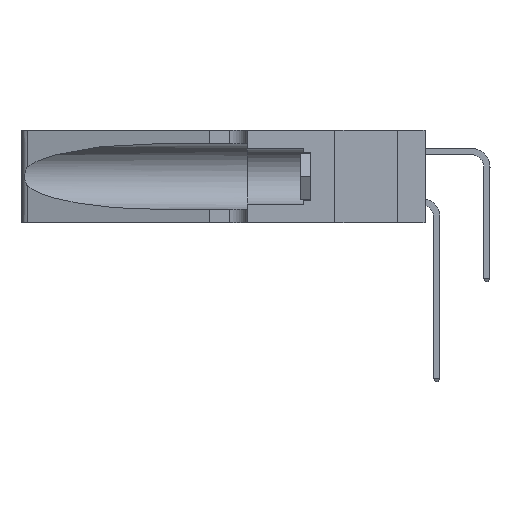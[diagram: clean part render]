
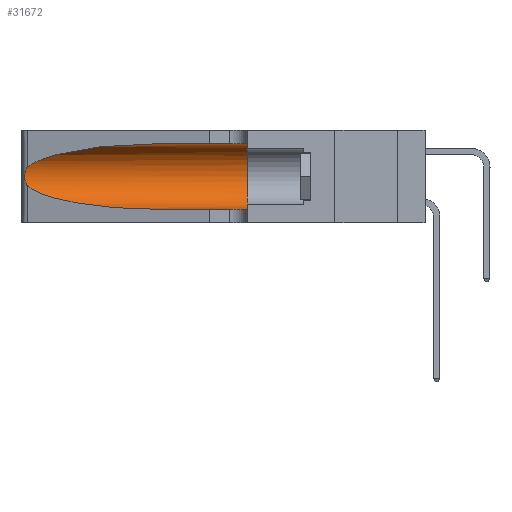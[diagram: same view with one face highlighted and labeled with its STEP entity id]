
A CAD part, left-side view. The second image highlights one B-rep face of the part: STEP entity #31672.
In plain terms, the highlighted cylindrical face has radius 3.308 mm (diameter 6.617 mm), a partial arc.
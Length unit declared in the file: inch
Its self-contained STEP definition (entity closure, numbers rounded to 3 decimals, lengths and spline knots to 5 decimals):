
#362 = CARTESIAN_POINT ( 'NONE',  ( 0.26017, 1.23833, 0.17102 ) ) ;
#567 = EDGE_LOOP ( 'NONE', ( #5458, #7572, #2621, #29499, #17899, #40339 ) ) ;
#2184 = CARTESIAN_POINT ( 'NONE',  ( 0.1305, 1.61858, 0.31525 ) ) ;
#2621 = ORIENTED_EDGE ( 'NONE', *, *, #37447, .T. ) ;
#4915 = CARTESIAN_POINT ( 'NONE',  ( 0.2373, 1.15595, 0.08982 ) ) ;
#5210 = CARTESIAN_POINT ( 'NONE',  ( 0.25487, 1.22718, 0.22369 ) ) ;
#5458 = ORIENTED_EDGE ( 'NONE', *, *, #31638, .T. ) ;
#5500 = CARTESIAN_POINT ( 'NONE',  ( 0.25555, 1.22994, 0.2215 ) ) ;
#5758 = CARTESIAN_POINT ( 'NONE',  ( 0.1305, 0.72297, 0.05475 ) ) ;
#5780 = CARTESIAN_POINT ( 'NONE',  ( 0.25487, 1.22718, 0.14631 ) ) ;
#6291 = VERTEX_POINT ( 'NONE', #24613 ) ;
#6397 = VERTEX_POINT ( 'NONE', #15946 ) ;
#7291 = CARTESIAN_POINT ( 'NONE',  ( 0.25487, 1.22718, 0.22369 ) ) ;
#7572 = ORIENTED_EDGE ( 'NONE', *, *, #22277, .T. ) ;
#8047 = DIRECTION ( 'NONE',  ( 0., -1., 0. ) ) ;
#8286 = DIRECTION ( 'NONE',  ( 0., 0., 1. ) ) ;
#8393 = CARTESIAN_POINT ( 'NONE',  ( 0.1305, 0.72297, 0.05475 ) ) ;
#8981 = CARTESIAN_POINT ( 'NONE',  ( 0.25854, 1.2359, 0.20912 ) ) ;
#10666 = CARTESIAN_POINT ( 'NONE',  ( 0.1305, 1.61858, 0.185 ) ) ;
#13302 = CARTESIAN_POINT ( 'NONE',  ( 0.25555, 1.22993, 0.14849 ) ) ;
#13354 = VECTOR ( 'NONE', #18808, 39.37008 ) ;
#13416 = VECTOR ( 'NONE', #8047, 39.37008 ) ;
#13711 = CARTESIAN_POINT ( 'NONE',  ( 0.25856, 1.23593, 0.16098 ) ) ;
#13867 = CARTESIAN_POINT ( 'NONE',  ( 0.25639, 1.23186, 0.15144 ) ) ;
#13980 = DIRECTION ( 'NONE',  ( 0., 0., -1. ) ) ;
#14607 = CARTESIAN_POINT ( 'NONE',  ( 0.1305, 0.35, 0.05475 ) ) ;
#15946 = CARTESIAN_POINT ( 'NONE',  ( 0.25487, 1.22718, 0.22369 ) ) ;
#16244 = EDGE_CURVE ( 'NONE', #22310, #40603, #24542, .T. ) ;
#17899 = ORIENTED_EDGE ( 'NONE', *, *, #16244, .F. ) ;
#17975 = CARTESIAN_POINT ( 'NONE',  ( 0.1305, 0.35, 0.185 ) ) ;
#18808 = DIRECTION ( 'NONE',  ( 0., -1., 0. ) ) ;
#19439 = AXIS2_PLACEMENT_3D ( 'NONE', #17975, #31708, #8286 ) ;
#19561 = EDGE_CURVE ( 'NONE', #21474, #40603, #24217, .T. ) ;
#19848 =( BOUNDED_CURVE ( )  B_SPLINE_CURVE ( 3, ( #37984, #4915, #28458, #8393 ),
 .UNSPECIFIED., .F., .T. ) 
 B_SPLINE_CURVE_WITH_KNOTS ( ( 4, 4 ),
 ( 3.44316, 4.71239 ),
 .UNSPECIFIED. ) 
 CURVE ( )  GEOMETRIC_REPRESENTATION_ITEM ( )  RATIONAL_B_SPLINE_CURVE ( ( 1., 0.87, 0.87, 1. ) ) 
 REPRESENTATION_ITEM ( '' )  );
#20047 = CARTESIAN_POINT ( 'NONE',  ( 0.26075, 1.23896, 0.178 ) ) ;
#21474 = VERTEX_POINT ( 'NONE', #5758 ) ;
#22277 = EDGE_CURVE ( 'NONE', #6397, #22812, #31537, .T. ) ;
#22310 = VERTEX_POINT ( 'NONE', #40669 ) ;
#22812 = VERTEX_POINT ( 'NONE', #5780 ) ;
#24217 = LINE ( 'NONE', #24340, #13416 ) ;
#24340 = CARTESIAN_POINT ( 'NONE',  ( 0.1305, 1.61858, 0.05475 ) ) ;
#24542 = CIRCLE ( 'NONE', #19439, 0.13025 ) ;
#24613 = CARTESIAN_POINT ( 'NONE',  ( 0.1305, 0.72297, 0.31525 ) ) ;
#25415 = CARTESIAN_POINT ( 'NONE',  ( 0.25787, 1.23484, 0.2124 ) ) ;
#27126 = EDGE_CURVE ( 'NONE', #6291, #22310, #38685, .T. ) ;
#27361 = CARTESIAN_POINT ( 'NONE',  ( 0.2373, 1.15595, 0.28018 ) ) ;
#28458 = CARTESIAN_POINT ( 'NONE',  ( 0.18966, 0.96281, 0.05475 ) ) ;
#28746 = CARTESIAN_POINT ( 'NONE',  ( 0.26018, 1.23835, 0.19895 ) ) ;
#29499 = ORIENTED_EDGE ( 'NONE', *, *, #19561, .T. ) ;
#30701 = AXIS2_PLACEMENT_3D ( 'NONE', #10666, #37191, #13980 ) ;
#31537 = B_SPLINE_CURVE_WITH_KNOTS ( 'NONE', 3,
 ( #5210, #5500, #41892, #25415, #8981, #28746, #38702, #20047, #362, #13711, #40092, #13867, #13302, #34025 ),
 .UNSPECIFIED., .F., .F.,
 ( 4, 2, 2, 2, 2, 2, 4 ),
 ( 0., 0.00027, 0.00053, 0.00107, 0.0016, 0.00187, 0.00214 ),
 .UNSPECIFIED. ) ;
#31638 = EDGE_CURVE ( 'NONE', #6291, #6397, #35230, .T. ) ;
#31672 = ADVANCED_FACE ( 'NONE', ( #40396 ), #36809, .F. ) ;
#31708 = DIRECTION ( 'NONE',  ( 0., 1., 0. ) ) ;
#32471 = CARTESIAN_POINT ( 'NONE',  ( 0.1305, 0.72297, 0.31525 ) ) ;
#34025 = CARTESIAN_POINT ( 'NONE',  ( 0.25487, 1.22718, 0.14631 ) ) ;
#35230 =( BOUNDED_CURVE ( )  B_SPLINE_CURVE ( 3, ( #32471, #35768, #27361, #7291 ),
 .UNSPECIFIED., .F., .T. ) 
 B_SPLINE_CURVE_WITH_KNOTS ( ( 4, 4 ),
 ( 1.5708, 2.84003 ),
 .UNSPECIFIED. ) 
 CURVE ( )  GEOMETRIC_REPRESENTATION_ITEM ( )  RATIONAL_B_SPLINE_CURVE ( ( 1., 0.87, 0.87, 1. ) ) 
 REPRESENTATION_ITEM ( '' )  );
#35768 = CARTESIAN_POINT ( 'NONE',  ( 0.18966, 0.96281, 0.31525 ) ) ;
#36809 = CYLINDRICAL_SURFACE ( 'NONE', #30701, 0.13025 ) ;
#37191 = DIRECTION ( 'NONE',  ( 0., -1., 0. ) ) ;
#37447 = EDGE_CURVE ( 'NONE', #22812, #21474, #19848, .T. ) ;
#37984 = CARTESIAN_POINT ( 'NONE',  ( 0.25487, 1.22718, 0.14631 ) ) ;
#38685 = LINE ( 'NONE', #2184, #13354 ) ;
#38702 = CARTESIAN_POINT ( 'NONE',  ( 0.26075, 1.23896, 0.19203 ) ) ;
#40092 = CARTESIAN_POINT ( 'NONE',  ( 0.25789, 1.23486, 0.15765 ) ) ;
#40339 = ORIENTED_EDGE ( 'NONE', *, *, #27126, .F. ) ;
#40396 = FACE_OUTER_BOUND ( 'NONE', #567, .T. ) ;
#40603 = VERTEX_POINT ( 'NONE', #14607 ) ;
#40669 = CARTESIAN_POINT ( 'NONE',  ( 0.1305, 0.35, 0.31525 ) ) ;
#41892 = CARTESIAN_POINT ( 'NONE',  ( 0.25639, 1.23184, 0.21858 ) ) ;
